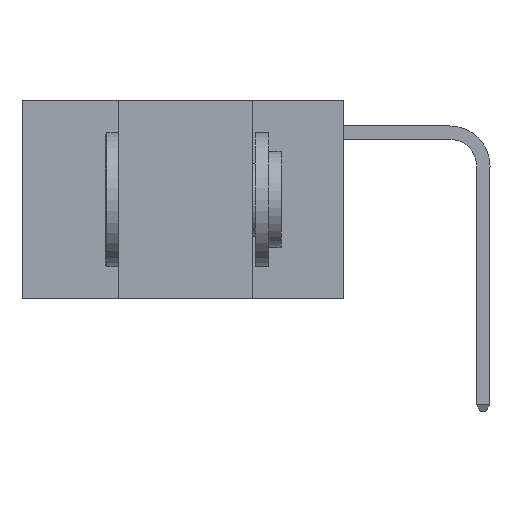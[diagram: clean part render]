
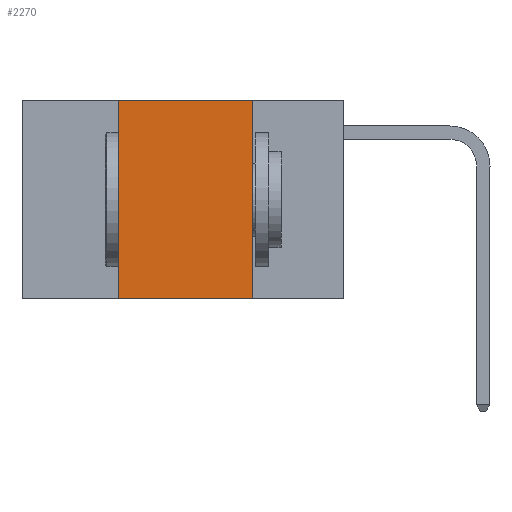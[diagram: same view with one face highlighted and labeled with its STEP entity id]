
A CAD part, left-side view. The second image highlights one B-rep face of the part: STEP entity #2270.
In plain terms, the highlighted planar face has unit normal (-1, 0, 0).
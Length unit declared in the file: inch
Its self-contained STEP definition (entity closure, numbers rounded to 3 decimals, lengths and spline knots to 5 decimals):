
#310 = VERTEX_POINT ( 'NONE', #12530 ) ;
#431 = EDGE_LOOP ( 'NONE', ( #1504, #1553, #1566, #1661 ) ) ;
#996 = AXIS2_PLACEMENT_3D ( 'NONE', #2768, #2811, #2595 ) ;
#1313 = CARTESIAN_POINT ( 'NONE',  ( 0., 0.42, 0. ) ) ;
#1501 = EDGE_CURVE ( 'NONE', #4620, #5136, #5226, .T. ) ;
#1504 = ORIENTED_EDGE ( 'NONE', *, *, #10189, .F. ) ;
#1553 = ORIENTED_EDGE ( 'NONE', *, *, #1501, .F. ) ;
#1566 = ORIENTED_EDGE ( 'NONE', *, *, #10369, .F. ) ;
#1661 = ORIENTED_EDGE ( 'NONE', *, *, #11894, .T. ) ;
#1825 = VERTEX_POINT ( 'NONE', #5032 ) ;
#2104 = DIRECTION ( 'NONE',  ( 0., -1., 0. ) ) ;
#2270 = ADVANCED_FACE ( 'NONE', ( #3106 ), #2640, .F. ) ;
#2462 = CARTESIAN_POINT ( 'NONE',  ( 0., 0.17, 0. ) ) ;
#2595 = DIRECTION ( 'NONE',  ( 0., 0., -1. ) ) ;
#2640 = PLANE ( 'NONE',  #996 ) ;
#2768 = CARTESIAN_POINT ( 'NONE',  ( 0., 0.6, 0. ) ) ;
#2811 = DIRECTION ( 'NONE',  ( 1., 0., 0. ) ) ;
#3106 = FACE_OUTER_BOUND ( 'NONE', #431, .T. ) ;
#3428 = VECTOR ( 'NONE', #6759, 39.37008 ) ;
#4620 = VERTEX_POINT ( 'NONE', #1313 ) ;
#5032 = CARTESIAN_POINT ( 'NONE',  ( 0., 0.17, -0.37 ) ) ;
#5136 = VERTEX_POINT ( 'NONE', #2462 ) ;
#5226 = LINE ( 'NONE', #6803, #3428 ) ;
#6759 = DIRECTION ( 'NONE',  ( 0., -1., 0. ) ) ;
#6803 = CARTESIAN_POINT ( 'NONE',  ( 0., 0.6, 0. ) ) ;
#7180 = CARTESIAN_POINT ( 'NONE',  ( 0., 0.6, -0.37 ) ) ;
#7238 = VECTOR ( 'NONE', #10321, 39.37008 ) ;
#8660 = LINE ( 'NONE', #7180, #10528 ) ;
#8846 = DIRECTION ( 'NONE',  ( 0., 0., -1. ) ) ;
#9898 = CARTESIAN_POINT ( 'NONE',  ( 0., 0.17, 0. ) ) ;
#10189 = EDGE_CURVE ( 'NONE', #5136, #1825, #13109, .T. ) ;
#10321 = DIRECTION ( 'NONE',  ( 0., 0., 1. ) ) ;
#10369 = EDGE_CURVE ( 'NONE', #310, #4620, #10387, .T. ) ;
#10387 = LINE ( 'NONE', #12284, #7238 ) ;
#10528 = VECTOR ( 'NONE', #2104, 39.37008 ) ;
#11894 = EDGE_CURVE ( 'NONE', #310, #1825, #8660, .T. ) ;
#12284 = CARTESIAN_POINT ( 'NONE',  ( 0., 0.42, 0. ) ) ;
#12530 = CARTESIAN_POINT ( 'NONE',  ( 0., 0.42, -0.37 ) ) ;
#12797 = VECTOR ( 'NONE', #8846, 39.37008 ) ;
#13109 = LINE ( 'NONE', #9898, #12797 ) ;
